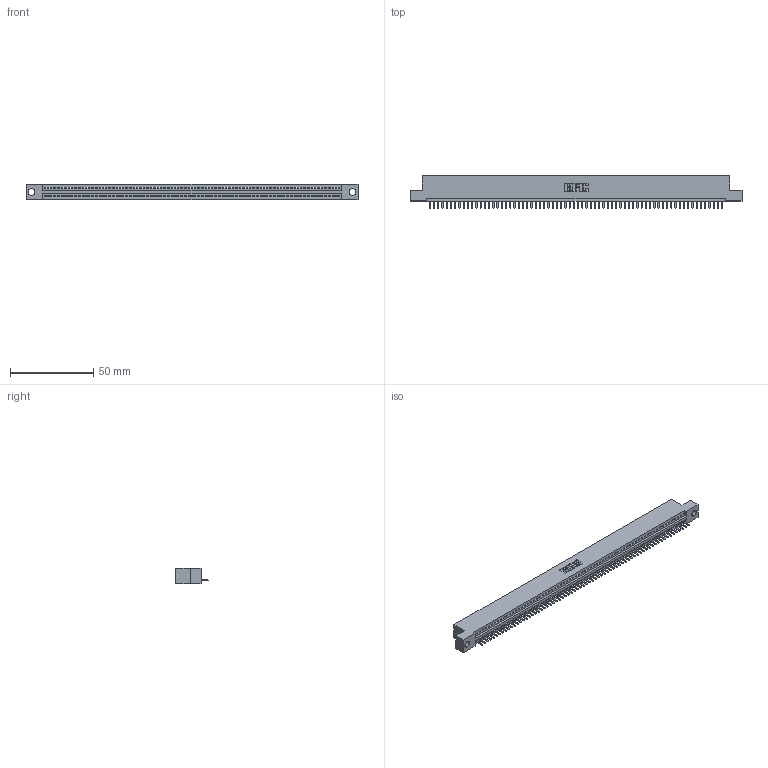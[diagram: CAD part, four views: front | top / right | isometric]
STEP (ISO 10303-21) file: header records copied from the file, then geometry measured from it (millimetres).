
FILE_DESCRIPTION (( 'STEP AP203' ), '1' );
FILE_NAME ('395-070-520-104.STEP', '2018-11-26T13:16:02', ( '' ), ( '' ), 'SwSTEP 2.0', 'SolidWorks 2016', '' );
FILE_SCHEMA (( 'CONFIG_CONTROL_DESIGN' ));
Length unit declared in the file: inch
Products named in the file (3): 345 Part_Flush Mounting Lugs - 0.156 Dia-TH; 345-292-001_345-293-120; 395-070-520-104
Assembly tree (71 placements, depth 2):
  395-070-520-104
    345 Part_Flush Mounting Lugs - 0.156 Dia-TH
    345-292-001_345-293-120  x70
Bounding box: 199.01 x 19.68 x 9.4 mm (x, y, z)
Volume: 18842.2 mm3; surface area: 24570.2 mm2
Topology: 71 solids, 71 shells, 4466 faces, 13221 edges, 8626 vertices
Faces by surface type: plane 3020, cylinder 1446
Entity records: 49031 total; most frequent: CARTESIAN_POINT 8510, ORIENTED_EDGE 8502, DIRECTION 7379, EDGE_CURVE 4251, VECTOR 3835, LINE 3835, VERTEX_POINT 2830, AXIS2_PLACEMENT_3D 1772
